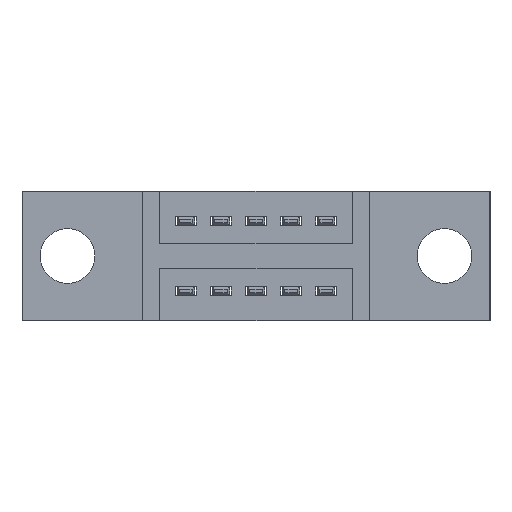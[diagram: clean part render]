
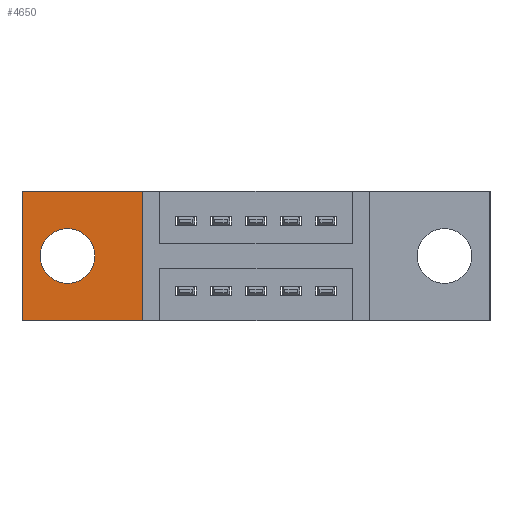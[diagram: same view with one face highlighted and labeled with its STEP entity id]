
A CAD part, front view. The second image highlights one B-rep face of the part: STEP entity #4650.
In plain terms, the highlighted planar face has unit normal (0, -1, 0).
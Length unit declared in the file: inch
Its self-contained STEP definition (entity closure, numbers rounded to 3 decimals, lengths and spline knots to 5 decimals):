
#310 = CARTESIAN_POINT ( 'NONE',  ( 0.3425, 0.17, -0.37 ) ) ;
#509 = VECTOR ( 'NONE', #1589, 39.37008 ) ;
#726 = LINE ( 'NONE', #3633, #7884 ) ;
#868 = EDGE_CURVE ( 'NONE', #1200, #1659, #6703, .T. ) ;
#904 = VERTEX_POINT ( 'NONE', #310 ) ;
#1016 = DIRECTION ( 'NONE',  ( 0., -1., 0. ) ) ;
#1176 = CARTESIAN_POINT ( 'NONE',  ( 0.13, 0.17, -0.107 ) ) ;
#1200 = VERTEX_POINT ( 'NONE', #1176 ) ;
#1328 = DIRECTION ( 'NONE',  ( 0., -1., 0. ) ) ;
#1527 = PLANE ( 'NONE',  #1623 ) ;
#1569 = DIRECTION ( 'NONE',  ( 0., 0., -1. ) ) ;
#1589 = DIRECTION ( 'NONE',  ( 0., 0., 1. ) ) ;
#1623 = AXIS2_PLACEMENT_3D ( 'NONE', #2476, #1328, #1569 ) ;
#1658 = CARTESIAN_POINT ( 'NONE',  ( 0., 0.17, 0. ) ) ;
#1659 = VERTEX_POINT ( 'NONE', #7852 ) ;
#1920 = ORIENTED_EDGE ( 'NONE', *, *, #8685, .T. ) ;
#1942 = CIRCLE ( 'NONE', #6982, 0.078 ) ;
#2353 = VERTEX_POINT ( 'NONE', #6270 ) ;
#2409 = DIRECTION ( 'NONE',  ( -1., 0., 0. ) ) ;
#2476 = CARTESIAN_POINT ( 'NONE',  ( 0., 0.17, -0.37 ) ) ;
#2941 = CARTESIAN_POINT ( 'NONE',  ( 0.13, 0.17, -0.185 ) ) ;
#2997 = LINE ( 'NONE', #7438, #6687 ) ;
#3095 = VERTEX_POINT ( 'NONE', #1658 ) ;
#3119 = VECTOR ( 'NONE', #2409, 39.37008 ) ;
#3268 = ORIENTED_EDGE ( 'NONE', *, *, #7540, .T. ) ;
#3385 = CARTESIAN_POINT ( 'NONE',  ( 0.3425, 0.17, 0. ) ) ;
#3436 = EDGE_LOOP ( 'NONE', ( #6531, #4628 ) ) ;
#3556 = EDGE_CURVE ( 'NONE', #2353, #904, #726, .T. ) ;
#3588 = DIRECTION ( 'NONE',  ( 1., 0., 0. ) ) ;
#3633 = CARTESIAN_POINT ( 'NONE',  ( 0., 0.17, -0.37 ) ) ;
#3831 = CARTESIAN_POINT ( 'NONE',  ( 0.3425, 0.17, 0. ) ) ;
#4603 = EDGE_CURVE ( 'NONE', #1659, #1200, #1942, .T. ) ;
#4628 = ORIENTED_EDGE ( 'NONE', *, *, #4603, .F. ) ;
#4650 = ADVANCED_FACE ( 'NONE', ( #8523, #5358 ), #1527, .T. ) ;
#5267 = ORIENTED_EDGE ( 'NONE', *, *, #3556, .T. ) ;
#5358 = FACE_OUTER_BOUND ( 'NONE', #5859, .T. ) ;
#5859 = EDGE_LOOP ( 'NONE', ( #1920, #5267, #3268, #7412 ) ) ;
#6270 = CARTESIAN_POINT ( 'NONE',  ( 0., 0.17, -0.37 ) ) ;
#6531 = ORIENTED_EDGE ( 'NONE', *, *, #868, .F. ) ;
#6687 = VECTOR ( 'NONE', #8051, 39.37008 ) ;
#6703 = CIRCLE ( 'NONE', #6945, 0.078 ) ;
#6945 = AXIS2_PLACEMENT_3D ( 'NONE', #2941, #1016, #8793 ) ;
#6982 = AXIS2_PLACEMENT_3D ( 'NONE', #7898, #7919, #7534 ) ;
#7412 = ORIENTED_EDGE ( 'NONE', *, *, #8433, .T. ) ;
#7438 = CARTESIAN_POINT ( 'NONE',  ( 0., 0.17, 0. ) ) ;
#7534 = DIRECTION ( 'NONE',  ( 0., 0., -1. ) ) ;
#7540 = EDGE_CURVE ( 'NONE', #904, #8688, #7882, .T. ) ;
#7852 = CARTESIAN_POINT ( 'NONE',  ( 0.13, 0.17, -0.263 ) ) ;
#7862 = CARTESIAN_POINT ( 'NONE',  ( 0., 0.17, 0. ) ) ;
#7882 = LINE ( 'NONE', #3831, #509 ) ;
#7884 = VECTOR ( 'NONE', #3588, 39.37008 ) ;
#7898 = CARTESIAN_POINT ( 'NONE',  ( 0.13, 0.17, -0.185 ) ) ;
#7919 = DIRECTION ( 'NONE',  ( 0., -1., 0. ) ) ;
#8051 = DIRECTION ( 'NONE',  ( 0., 0., -1. ) ) ;
#8433 = EDGE_CURVE ( 'NONE', #8688, #3095, #8434, .T. ) ;
#8434 = LINE ( 'NONE', #7862, #3119 ) ;
#8523 = FACE_BOUND ( 'NONE', #3436, .T. ) ;
#8685 = EDGE_CURVE ( 'NONE', #3095, #2353, #2997, .T. ) ;
#8688 = VERTEX_POINT ( 'NONE', #3385 ) ;
#8793 = DIRECTION ( 'NONE',  ( 0., 0., -1. ) ) ;
